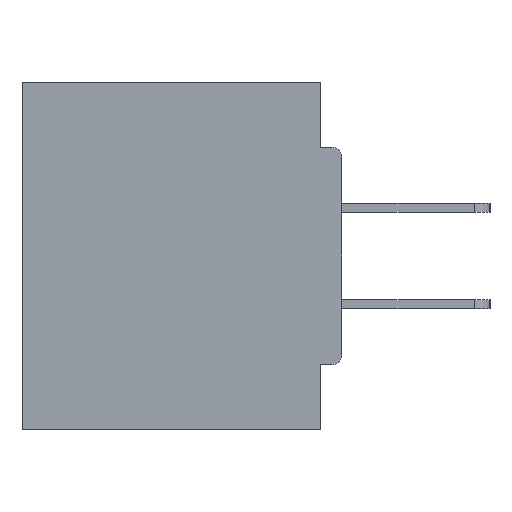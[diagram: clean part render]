
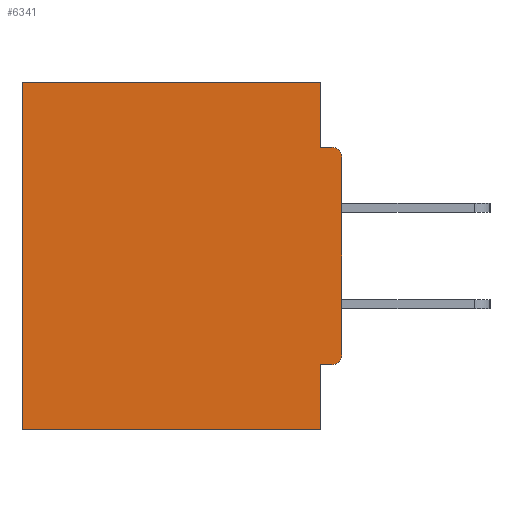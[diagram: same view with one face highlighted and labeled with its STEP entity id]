
A CAD part, left-side view. The second image highlights one B-rep face of the part: STEP entity #6341.
In plain terms, the highlighted planar face has unit normal (-1, 0, 0).
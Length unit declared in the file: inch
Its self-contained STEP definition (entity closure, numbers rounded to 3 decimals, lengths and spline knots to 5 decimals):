
#1011 = CARTESIAN_POINT ( 'NONE',  ( 0.298, 0., 0. ) ) ;
#1354 = VECTOR ( 'NONE', #7142, 39.37008 ) ;
#2383 = EDGE_CURVE ( 'NONE', #38155, #7358, #32143, .T. ) ;
#2483 = DIRECTION ( 'NONE',  ( 0., 1., 0. ) ) ;
#2619 = CARTESIAN_POINT ( 'NONE',  ( 0.298, 0.015, -0.4065 ) ) ;
#2951 = CARTESIAN_POINT ( 'NONE',  ( 0.298, 0.031, -0.5 ) ) ;
#3047 = VERTEX_POINT ( 'NONE', #2619 ) ;
#3065 = EDGE_CURVE ( 'NONE', #9413, #17037, #20691, .T. ) ;
#3361 = ORIENTED_EDGE ( 'NONE', *, *, #3065, .F. ) ;
#3711 = CARTESIAN_POINT ( 'NONE',  ( 0.298, 0., 0. ) ) ;
#3731 = VERTEX_POINT ( 'NONE', #18083 ) ;
#4117 = VERTEX_POINT ( 'NONE', #29331 ) ;
#4202 = CARTESIAN_POINT ( 'NONE',  ( 0.298, 0., -0.1085 ) ) ;
#5083 = CARTESIAN_POINT ( 'NONE',  ( 0.298, 0.031, 0. ) ) ;
#5085 = VECTOR ( 'NONE', #7730, 39.37008 ) ;
#5708 = FACE_OUTER_BOUND ( 'NONE', #31304, .T. ) ;
#6331 = DIRECTION ( 'NONE',  ( -1., 0., 0. ) ) ;
#6341 = ADVANCED_FACE ( 'NONE', ( #5708 ), #6627, .F. ) ;
#6413 = CARTESIAN_POINT ( 'NONE',  ( 0.298, 0.46, -0.5 ) ) ;
#6627 = PLANE ( 'NONE',  #34293 ) ;
#6969 = LINE ( 'NONE', #3711, #30700 ) ;
#7142 = DIRECTION ( 'NONE',  ( 0., 1., 0. ) ) ;
#7261 = CIRCLE ( 'NONE', #30877, 0.015 ) ;
#7358 = VERTEX_POINT ( 'NONE', #38444 ) ;
#7730 = DIRECTION ( 'NONE',  ( 0., -1., 0. ) ) ;
#9413 = VERTEX_POINT ( 'NONE', #26523 ) ;
#10398 = LINE ( 'NONE', #2951, #28447 ) ;
#11178 = DIRECTION ( 'NONE',  ( 0., 1., 0. ) ) ;
#11354 = EDGE_CURVE ( 'NONE', #3047, #4117, #7261, .T. ) ;
#11630 = DIRECTION ( 'NONE',  ( 0., 0., -1. ) ) ;
#12651 = VECTOR ( 'NONE', #2483, 39.37008 ) ;
#13602 = EDGE_CURVE ( 'NONE', #22019, #17037, #38988, .T. ) ;
#13883 = ORIENTED_EDGE ( 'NONE', *, *, #13602, .T. ) ;
#14220 = ORIENTED_EDGE ( 'NONE', *, *, #26202, .T. ) ;
#14745 = DIRECTION ( 'NONE',  ( -1., 0., 0. ) ) ;
#14919 = DIRECTION ( 'NONE',  ( 0., 0., -1. ) ) ;
#15004 = DIRECTION ( 'NONE',  ( 0., 0., -1. ) ) ;
#15164 = DIRECTION ( 'NONE',  ( 0., 0., -1. ) ) ;
#16027 = DIRECTION ( 'NONE',  ( 0., 0., -1. ) ) ;
#16165 = VERTEX_POINT ( 'NONE', #4202 ) ;
#16214 = EDGE_CURVE ( 'NONE', #34104, #22019, #17985, .T. ) ;
#16541 = EDGE_CURVE ( 'NONE', #34104, #38155, #10398, .T. ) ;
#17037 = VERTEX_POINT ( 'NONE', #6413 ) ;
#17833 = CARTESIAN_POINT ( 'NONE',  ( 0.298, 0.46, 0. ) ) ;
#17914 = CARTESIAN_POINT ( 'NONE',  ( 0.298, 0.015, -0.3915 ) ) ;
#17985 = LINE ( 'NONE', #1011, #1354 ) ;
#18083 = CARTESIAN_POINT ( 'NONE',  ( 0.298, 0.031, -0.4065 ) ) ;
#18485 = CARTESIAN_POINT ( 'NONE',  ( 0.298, 0.031, -0.0935 ) ) ;
#18703 = VECTOR ( 'NONE', #21451, 39.37008 ) ;
#18948 = ORIENTED_EDGE ( 'NONE', *, *, #16541, .F. ) ;
#19114 = DIRECTION ( 'NONE',  ( 0., 0., -1. ) ) ;
#19877 = EDGE_CURVE ( 'NONE', #3047, #3731, #22548, .T. ) ;
#20016 = ORIENTED_EDGE ( 'NONE', *, *, #11354, .T. ) ;
#20096 = ORIENTED_EDGE ( 'NONE', *, *, #28461, .F. ) ;
#20583 = EDGE_CURVE ( 'NONE', #3731, #9413, #23430, .T. ) ;
#20691 = LINE ( 'NONE', #23840, #12651 ) ;
#21451 = DIRECTION ( 'NONE',  ( 0., 0., -1. ) ) ;
#21575 = CARTESIAN_POINT ( 'NONE',  ( 0.298, 0.015, -0.1085 ) ) ;
#22019 = VERTEX_POINT ( 'NONE', #25055 ) ;
#22548 = LINE ( 'NONE', #23485, #38610 ) ;
#23137 = ORIENTED_EDGE ( 'NONE', *, *, #2383, .F. ) ;
#23430 = LINE ( 'NONE', #27567, #18703 ) ;
#23485 = CARTESIAN_POINT ( 'NONE',  ( 0.298, 0., -0.4065 ) ) ;
#23840 = CARTESIAN_POINT ( 'NONE',  ( 0.298, 0., -0.5 ) ) ;
#25055 = CARTESIAN_POINT ( 'NONE',  ( 0.298, 0.46, 0. ) ) ;
#25298 = VECTOR ( 'NONE', #11630, 39.37008 ) ;
#25815 = ORIENTED_EDGE ( 'NONE', *, *, #16214, .T. ) ;
#26202 = EDGE_CURVE ( 'NONE', #16165, #7358, #35578, .T. ) ;
#26523 = CARTESIAN_POINT ( 'NONE',  ( 0.298, 0.031, -0.5 ) ) ;
#27567 = CARTESIAN_POINT ( 'NONE',  ( 0.298, 0.031, -0.5 ) ) ;
#27868 = DIRECTION ( 'NONE',  ( 1., 0., 0. ) ) ;
#28000 = CARTESIAN_POINT ( 'NONE',  ( 0.298, 0., 0. ) ) ;
#28221 = ORIENTED_EDGE ( 'NONE', *, *, #19877, .F. ) ;
#28447 = VECTOR ( 'NONE', #15164, 39.37008 ) ;
#28461 = EDGE_CURVE ( 'NONE', #16165, #4117, #6969, .T. ) ;
#29331 = CARTESIAN_POINT ( 'NONE',  ( 0.298, 0., -0.3915 ) ) ;
#30700 = VECTOR ( 'NONE', #19114, 39.37008 ) ;
#30877 = AXIS2_PLACEMENT_3D ( 'NONE', #17914, #14745, #15004 ) ;
#31304 = EDGE_LOOP ( 'NONE', ( #14220, #23137, #18948, #25815, #13883, #3361, #34167, #28221, #20016, #20096 ) ) ;
#32143 = LINE ( 'NONE', #37284, #5085 ) ;
#34104 = VERTEX_POINT ( 'NONE', #5083 ) ;
#34167 = ORIENTED_EDGE ( 'NONE', *, *, #20583, .F. ) ;
#34293 = AXIS2_PLACEMENT_3D ( 'NONE', #28000, #27868, #16027 ) ;
#34525 = AXIS2_PLACEMENT_3D ( 'NONE', #21575, #6331, #14919 ) ;
#35578 = CIRCLE ( 'NONE', #34525, 0.015 ) ;
#37284 = CARTESIAN_POINT ( 'NONE',  ( 0.298, 0., -0.0935 ) ) ;
#38155 = VERTEX_POINT ( 'NONE', #18485 ) ;
#38444 = CARTESIAN_POINT ( 'NONE',  ( 0.298, 0.015, -0.0935 ) ) ;
#38610 = VECTOR ( 'NONE', #11178, 39.37008 ) ;
#38988 = LINE ( 'NONE', #17833, #25298 ) ;
